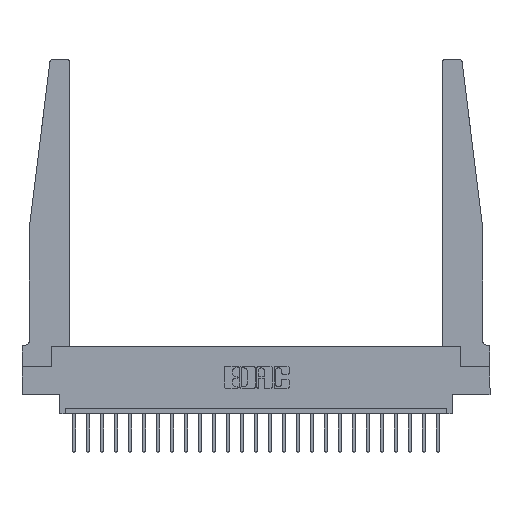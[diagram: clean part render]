
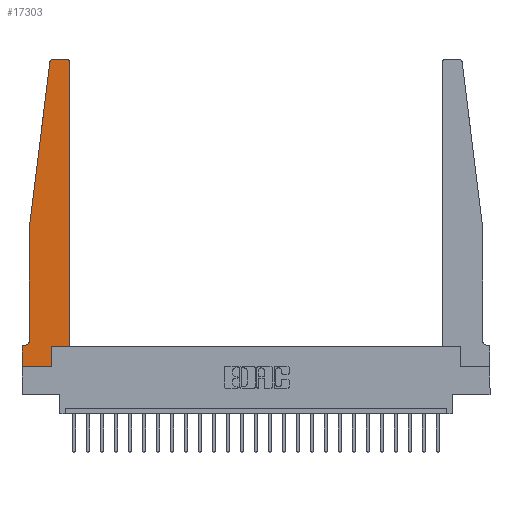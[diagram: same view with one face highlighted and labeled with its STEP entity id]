
A CAD part, top view. The second image highlights one B-rep face of the part: STEP entity #17303.
In plain terms, the highlighted planar face has unit normal (0, 0, 1).
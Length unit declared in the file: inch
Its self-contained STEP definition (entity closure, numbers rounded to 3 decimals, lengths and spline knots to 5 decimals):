
#150 = DIRECTION ( 'NONE',  ( 0., -1., 0. ) ) ;
#171 = EDGE_CURVE ( 'NONE', #12236, #22841, #21401, .T. ) ;
#209 = AXIS2_PLACEMENT_3D ( 'NONE', #335, #22909, #11660 ) ;
#297 = EDGE_CURVE ( 'NONE', #6960, #16735, #8984, .T. ) ;
#335 = CARTESIAN_POINT ( 'NONE',  ( 0.015, 0.2375, 0.37 ) ) ;
#423 = CARTESIAN_POINT ( 'NONE',  ( 0.2605, 0.18, 0.37 ) ) ;
#713 = DIRECTION ( 'NONE',  ( 1., 0., 0. ) ) ;
#732 = AXIS2_PLACEMENT_3D ( 'NONE', #21573, #6534, #10442 ) ;
#1340 = EDGE_CURVE ( 'NONE', #13553, #19460, #9887, .T. ) ;
#1395 = VECTOR ( 'NONE', #19362, 39.37008 ) ;
#1937 = ORIENTED_EDGE ( 'NONE', *, *, #1340, .T. ) ;
#2013 = EDGE_CURVE ( 'NONE', #15879, #23984, #21881, .T. ) ;
#2062 = LINE ( 'NONE', #20618, #5106 ) ;
#2213 = EDGE_CURVE ( 'NONE', #4805, #15879, #2600, .T. ) ;
#2600 = LINE ( 'NONE', #10040, #14434 ) ;
#3414 = ORIENTED_EDGE ( 'NONE', *, *, #15065, .T. ) ;
#3502 = DIRECTION ( 'NONE',  ( 0., -1., 0. ) ) ;
#3956 = VECTOR ( 'NONE', #150, 39.37008 ) ;
#4046 = LINE ( 'NONE', #22364, #3956 ) ;
#4462 = CIRCLE ( 'NONE', #209, 0.05 ) ;
#4764 = EDGE_CURVE ( 'NONE', #23984, #12236, #2062, .T. ) ;
#4805 = VERTEX_POINT ( 'NONE', #24048 ) ;
#4998 = ORIENTED_EDGE ( 'NONE', *, *, #8509, .T. ) ;
#5049 = CARTESIAN_POINT ( 'NONE',  ( 0.425, 0.18, 0.37 ) ) ;
#5106 = VECTOR ( 'NONE', #16810, 39.37008 ) ;
#5578 = EDGE_CURVE ( 'NONE', #8863, #4805, #6874, .T. ) ;
#5894 = DIRECTION ( 'NONE',  ( 1., 0., 0. ) ) ;
#6180 = DIRECTION ( 'NONE',  ( 0., 0., 1. ) ) ;
#6213 = ORIENTED_EDGE ( 'NONE', *, *, #2013, .T. ) ;
#6278 = VERTEX_POINT ( 'NONE', #19512 ) ;
#6534 = DIRECTION ( 'NONE',  ( 0., 0., 1. ) ) ;
#6692 = DIRECTION ( 'NONE',  ( 1., 0., 0. ) ) ;
#6856 = CARTESIAN_POINT ( 'NONE',  ( 0.24675, 2.72367, 0.37 ) ) ;
#6874 = LINE ( 'NONE', #5049, #10992 ) ;
#6960 = VERTEX_POINT ( 'NONE', #22765 ) ;
#7422 = AXIS2_PLACEMENT_3D ( 'NONE', #22763, #16995, #5894 ) ;
#8158 = CARTESIAN_POINT ( 'NONE',  ( 0.27653, 2.75, 0.37 ) ) ;
#8170 = CARTESIAN_POINT ( 'NONE',  ( 0., 0., 0.37 ) ) ;
#8509 = EDGE_CURVE ( 'NONE', #16735, #13747, #4462, .T. ) ;
#8863 = VERTEX_POINT ( 'NONE', #423 ) ;
#8984 = LINE ( 'NONE', #23640, #9330 ) ;
#9330 = VECTOR ( 'NONE', #3502, 39.37008 ) ;
#9745 = FACE_OUTER_BOUND ( 'NONE', #12426, .T. ) ;
#9887 = LINE ( 'NONE', #8170, #21436 ) ;
#10040 = CARTESIAN_POINT ( 'NONE',  ( 0.425, 0.18, 0.37 ) ) ;
#10268 = VECTOR ( 'NONE', #18344, 39.37008 ) ;
#10442 = DIRECTION ( 'NONE',  ( 1., 0., 0. ) ) ;
#10992 = VECTOR ( 'NONE', #21429, 39.37008 ) ;
#11149 = CARTESIAN_POINT ( 'NONE',  ( 0.065, 0.1875, 0.37 ) ) ;
#11362 = ORIENTED_EDGE ( 'NONE', *, *, #11410, .T. ) ;
#11410 = EDGE_CURVE ( 'NONE', #19460, #8863, #20300, .T. ) ;
#11660 = DIRECTION ( 'NONE',  ( -1., 0., 0. ) ) ;
#11932 = CARTESIAN_POINT ( 'NONE',  ( 0.065, 1.25, 0.37 ) ) ;
#11937 = CARTESIAN_POINT ( 'NONE',  ( 0., 0.1875, 0.37 ) ) ;
#12236 = VERTEX_POINT ( 'NONE', #8158 ) ;
#12426 = EDGE_LOOP ( 'NONE', ( #21563, #21721, #20137, #15077, #4998, #21256, #3414, #1937, #11362, #18280, #16238, #6213 ) ) ;
#12486 = CARTESIAN_POINT ( 'NONE',  ( 0.2605, 0.18, 0.37 ) ) ;
#12723 = CARTESIAN_POINT ( 'NONE',  ( 0.065, 0.2375, 0.37 ) ) ;
#12971 = DIRECTION ( 'NONE',  ( 0., 1., 0. ) ) ;
#13553 = VERTEX_POINT ( 'NONE', #19905 ) ;
#13747 = VERTEX_POINT ( 'NONE', #20646 ) ;
#14434 = VECTOR ( 'NONE', #17832, 39.37008 ) ;
#15065 = EDGE_CURVE ( 'NONE', #6278, #13553, #4046, .T. ) ;
#15077 = ORIENTED_EDGE ( 'NONE', *, *, #297, .T. ) ;
#15303 = CARTESIAN_POINT ( 'NONE',  ( 0.2605, 0., 0.37 ) ) ;
#15879 = VERTEX_POINT ( 'NONE', #23888 ) ;
#16238 = ORIENTED_EDGE ( 'NONE', *, *, #2213, .T. ) ;
#16735 = VERTEX_POINT ( 'NONE', #12723 ) ;
#16810 = DIRECTION ( 'NONE',  ( -1., 0., 0. ) ) ;
#16861 = LINE ( 'NONE', #11149, #10268 ) ;
#16995 = DIRECTION ( 'NONE',  ( 0., 0., 1. ) ) ;
#17303 = ADVANCED_FACE ( 'NONE', ( #9745 ), #19131, .T. ) ;
#17832 = DIRECTION ( 'NONE',  ( 0., 1., 0. ) ) ;
#18280 = ORIENTED_EDGE ( 'NONE', *, *, #5578, .T. ) ;
#18328 = LINE ( 'NONE', #11932, #1395 ) ;
#18344 = DIRECTION ( 'NONE',  ( -1., 0., 0. ) ) ;
#19131 = PLANE ( 'NONE',  #21954 ) ;
#19362 = DIRECTION ( 'NONE',  ( -0.122, -0.992, 0. ) ) ;
#19460 = VERTEX_POINT ( 'NONE', #15303 ) ;
#19512 = CARTESIAN_POINT ( 'NONE',  ( 0., 0.1875, 0.37 ) ) ;
#19845 = EDGE_CURVE ( 'NONE', #13747, #6278, #16861, .T. ) ;
#19905 = CARTESIAN_POINT ( 'NONE',  ( 0., 0., 0.37 ) ) ;
#20137 = ORIENTED_EDGE ( 'NONE', *, *, #21756, .T. ) ;
#20300 = LINE ( 'NONE', #12486, #22756 ) ;
#20618 = CARTESIAN_POINT ( 'NONE',  ( 0.25, 2.75, 0.37 ) ) ;
#20646 = CARTESIAN_POINT ( 'NONE',  ( 0.015, 0.1875, 0.37 ) ) ;
#21256 = ORIENTED_EDGE ( 'NONE', *, *, #19845, .T. ) ;
#21401 = CIRCLE ( 'NONE', #732, 0.03 ) ;
#21429 = DIRECTION ( 'NONE',  ( 1., 0., 0. ) ) ;
#21436 = VECTOR ( 'NONE', #6692, 39.37008 ) ;
#21563 = ORIENTED_EDGE ( 'NONE', *, *, #4764, .T. ) ;
#21573 = CARTESIAN_POINT ( 'NONE',  ( 0.27653, 2.72, 0.37 ) ) ;
#21721 = ORIENTED_EDGE ( 'NONE', *, *, #171, .T. ) ;
#21756 = EDGE_CURVE ( 'NONE', #22841, #6960, #18328, .T. ) ;
#21881 = CIRCLE ( 'NONE', #7422, 0.03 ) ;
#21896 = CARTESIAN_POINT ( 'NONE',  ( 0.395, 2.75, 0.37 ) ) ;
#21954 = AXIS2_PLACEMENT_3D ( 'NONE', #11937, #6180, #713 ) ;
#22364 = CARTESIAN_POINT ( 'NONE',  ( 0., 0., 0.37 ) ) ;
#22756 = VECTOR ( 'NONE', #12971, 39.37008 ) ;
#22763 = CARTESIAN_POINT ( 'NONE',  ( 0.395, 2.72, 0.37 ) ) ;
#22765 = CARTESIAN_POINT ( 'NONE',  ( 0.065, 1.25, 0.37 ) ) ;
#22841 = VERTEX_POINT ( 'NONE', #6856 ) ;
#22909 = DIRECTION ( 'NONE',  ( 0., 0., -1. ) ) ;
#23640 = CARTESIAN_POINT ( 'NONE',  ( 0.065, 1.25, 0.37 ) ) ;
#23888 = CARTESIAN_POINT ( 'NONE',  ( 0.425, 2.72, 0.37 ) ) ;
#23984 = VERTEX_POINT ( 'NONE', #21896 ) ;
#24048 = CARTESIAN_POINT ( 'NONE',  ( 0.425, 0.18, 0.37 ) ) ;
